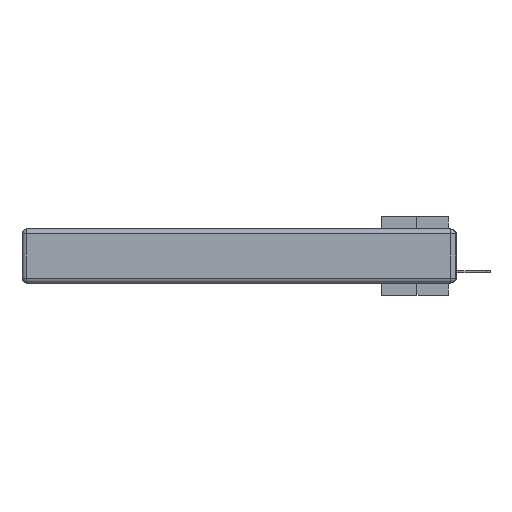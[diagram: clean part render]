
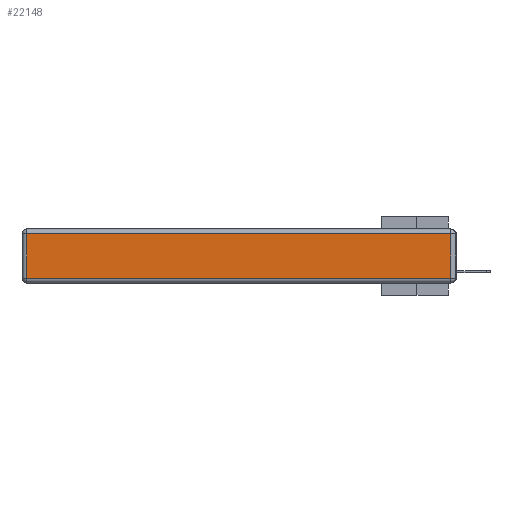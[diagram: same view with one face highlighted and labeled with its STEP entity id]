
A CAD part, left-side view. The second image highlights one B-rep face of the part: STEP entity #22148.
In plain terms, the highlighted planar face has unit normal (-1, 0, 0).
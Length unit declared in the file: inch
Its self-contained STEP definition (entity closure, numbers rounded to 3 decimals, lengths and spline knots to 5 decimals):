
#477 = VECTOR ( 'NONE', #1206, 39.37008 ) ;
#803 = VERTEX_POINT ( 'NONE', #30957 ) ;
#823 = AXIS2_PLACEMENT_3D ( 'NONE', #19399, #26758, #7540 ) ;
#1206 = DIRECTION ( 'NONE',  ( 0., -1., 0. ) ) ;
#2474 = VECTOR ( 'NONE', #11356, 39.37008 ) ;
#4703 = LINE ( 'NONE', #15702, #477 ) ;
#6644 = CARTESIAN_POINT ( 'NONE',  ( 0., 2.75, -0.03 ) ) ;
#6703 = EDGE_CURVE ( 'NONE', #22080, #6843, #4703, .T. ) ;
#6750 = DIRECTION ( 'NONE',  ( 0., 1., 0. ) ) ;
#6843 = VERTEX_POINT ( 'NONE', #27992 ) ;
#7540 = DIRECTION ( 'NONE',  ( 0., 0., 1. ) ) ;
#8867 = LINE ( 'NONE', #6644, #25964 ) ;
#9540 = CARTESIAN_POINT ( 'NONE',  ( 0., 2.72, -0.313 ) ) ;
#9999 = LINE ( 'NONE', #13761, #2474 ) ;
#11356 = DIRECTION ( 'NONE',  ( 0., 0., 1. ) ) ;
#12136 = FACE_OUTER_BOUND ( 'NONE', #27422, .T. ) ;
#13546 = VERTEX_POINT ( 'NONE', #18646 ) ;
#13683 = EDGE_CURVE ( 'NONE', #13546, #22080, #21257, .T. ) ;
#13761 = CARTESIAN_POINT ( 'NONE',  ( 0., 0.03, -0.343 ) ) ;
#14013 = CARTESIAN_POINT ( 'NONE',  ( 0., 2.72, -0.343 ) ) ;
#15702 = CARTESIAN_POINT ( 'NONE',  ( 0., 0., -0.313 ) ) ;
#16978 = PLANE ( 'NONE',  #823 ) ;
#18646 = CARTESIAN_POINT ( 'NONE',  ( 0., 2.72, -0.03 ) ) ;
#18961 = VECTOR ( 'NONE', #25632, 39.37008 ) ;
#19399 = CARTESIAN_POINT ( 'NONE',  ( 0., 0., -0.343 ) ) ;
#20218 = ORIENTED_EDGE ( 'NONE', *, *, #6703, .T. ) ;
#21257 = LINE ( 'NONE', #14013, #18961 ) ;
#22080 = VERTEX_POINT ( 'NONE', #9540 ) ;
#22148 = ADVANCED_FACE ( 'NONE', ( #12136 ), #16978, .T. ) ;
#22922 = EDGE_CURVE ( 'NONE', #6843, #803, #9999, .T. ) ;
#24509 = EDGE_CURVE ( 'NONE', #803, #13546, #8867, .T. ) ;
#24752 = ORIENTED_EDGE ( 'NONE', *, *, #13683, .T. ) ;
#24823 = ORIENTED_EDGE ( 'NONE', *, *, #24509, .T. ) ;
#25632 = DIRECTION ( 'NONE',  ( 0., 0., -1. ) ) ;
#25964 = VECTOR ( 'NONE', #6750, 39.37008 ) ;
#26758 = DIRECTION ( 'NONE',  ( -1., 0., 0. ) ) ;
#27422 = EDGE_LOOP ( 'NONE', ( #20218, #28201, #24823, #24752 ) ) ;
#27992 = CARTESIAN_POINT ( 'NONE',  ( 0., 0.03, -0.313 ) ) ;
#28201 = ORIENTED_EDGE ( 'NONE', *, *, #22922, .T. ) ;
#30957 = CARTESIAN_POINT ( 'NONE',  ( 0., 0.03, -0.03 ) ) ;
